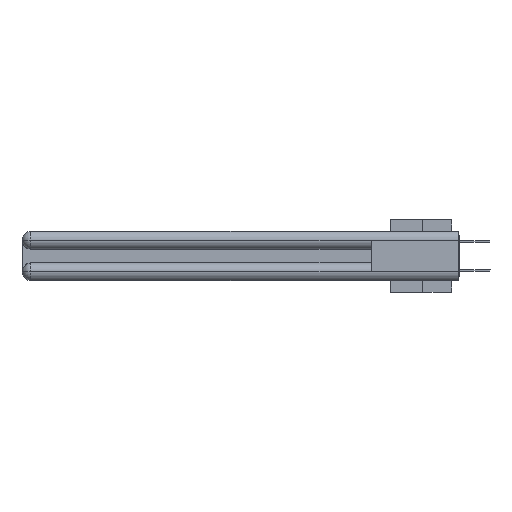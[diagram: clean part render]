
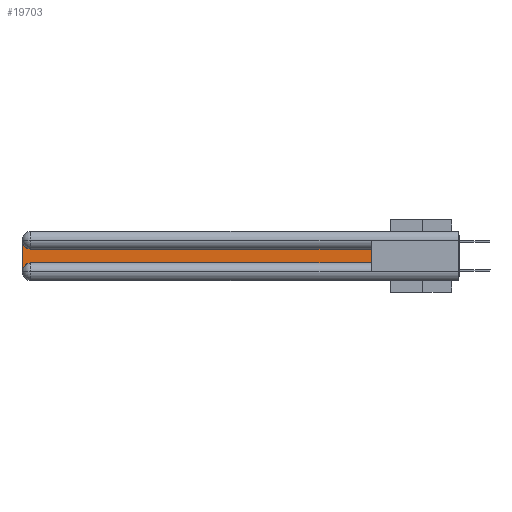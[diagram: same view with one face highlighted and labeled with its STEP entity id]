
A CAD part, left-side view. The second image highlights one B-rep face of the part: STEP entity #19703.
In plain terms, the highlighted planar face has unit normal (-1, 0, 0).
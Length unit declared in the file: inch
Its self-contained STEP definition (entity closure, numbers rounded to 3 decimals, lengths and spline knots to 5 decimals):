
#156 = DIRECTION ( 'NONE',  ( 1., 0., 0. ) ) ;
#2390 = CIRCLE ( 'NONE', #6401, 0.06 ) ;
#2912 = CARTESIAN_POINT ( 'NONE',  ( 0.075, 2.94, -0.0625 ) ) ;
#4606 = CARTESIAN_POINT ( 'NONE',  ( 0.075, 2.94, -0.2775 ) ) ;
#4840 = EDGE_CURVE ( 'NONE', #5301, #26955, #25053, .T. ) ;
#5238 = CARTESIAN_POINT ( 'NONE',  ( 0.075, 3., -0.1225 ) ) ;
#5301 = VERTEX_POINT ( 'NONE', #16665 ) ;
#5591 = AXIS2_PLACEMENT_3D ( 'NONE', #2912, #156, #28526 ) ;
#6158 = VECTOR ( 'NONE', #34325, 39.37008 ) ;
#6401 = AXIS2_PLACEMENT_3D ( 'NONE', #4606, #17427, #30210 ) ;
#6957 = ORIENTED_EDGE ( 'NONE', *, *, #10791, .T. ) ;
#7154 = DIRECTION ( 'NONE',  ( 0., 1., 0. ) ) ;
#7772 = CARTESIAN_POINT ( 'NONE',  ( 0.075, 0.6, -0.1225 ) ) ;
#8352 = CARTESIAN_POINT ( 'NONE',  ( 0.075, 0.6, -0.1225 ) ) ;
#8424 = CARTESIAN_POINT ( 'NONE',  ( 0.075, 2.94, -0.2175 ) ) ;
#8787 = DIRECTION ( 'NONE',  ( 0., 0., 1. ) ) ;
#10519 = LINE ( 'NONE', #7772, #22554 ) ;
#10764 = CARTESIAN_POINT ( 'NONE',  ( 0.075, 0.6, -0.2175 ) ) ;
#10791 = EDGE_CURVE ( 'NONE', #16378, #18903, #31024, .T. ) ;
#11516 = ORIENTED_EDGE ( 'NONE', *, *, #13961, .T. ) ;
#11784 = DIRECTION ( 'NONE',  ( 0., 0., -1. ) ) ;
#12517 = EDGE_LOOP ( 'NONE', ( #29094, #17004, #21422, #11516, #39699, #6957 ) ) ;
#13961 = EDGE_CURVE ( 'NONE', #41506, #39748, #2390, .T. ) ;
#15128 = FACE_OUTER_BOUND ( 'NONE', #12517, .T. ) ;
#16378 = VERTEX_POINT ( 'NONE', #10764 ) ;
#16665 = CARTESIAN_POINT ( 'NONE',  ( 0.075, 2.94, -0.1225 ) ) ;
#16806 = EDGE_CURVE ( 'NONE', #18903, #5301, #10519, .T. ) ;
#17004 = ORIENTED_EDGE ( 'NONE', *, *, #4840, .T. ) ;
#17427 = DIRECTION ( 'NONE',  ( 1., 0., 0. ) ) ;
#17859 = DIRECTION ( 'NONE',  ( 1., 0., 0. ) ) ;
#18283 = LINE ( 'NONE', #24157, #18512 ) ;
#18512 = VECTOR ( 'NONE', #11784, 39.37008 ) ;
#18903 = VERTEX_POINT ( 'NONE', #8352 ) ;
#19703 = ADVANCED_FACE ( 'NONE', ( #15128 ), #30845, .F. ) ;
#20860 = EDGE_CURVE ( 'NONE', #39748, #16378, #41042, .T. ) ;
#21422 = ORIENTED_EDGE ( 'NONE', *, *, #39660, .T. ) ;
#22264 = VECTOR ( 'NONE', #8787, 39.37008 ) ;
#22554 = VECTOR ( 'NONE', #7154, 39.37008 ) ;
#23931 = DIRECTION ( 'NONE',  ( 0., 0., -1. ) ) ;
#24157 = CARTESIAN_POINT ( 'NONE',  ( 0.075, 3., -0.2175 ) ) ;
#25053 = CIRCLE ( 'NONE', #5591, 0.06 ) ;
#26955 = VERTEX_POINT ( 'NONE', #33388 ) ;
#28099 = CARTESIAN_POINT ( 'NONE',  ( 0.075, 0.6, -0.2175 ) ) ;
#28526 = DIRECTION ( 'NONE',  ( 0., 0., -1. ) ) ;
#29094 = ORIENTED_EDGE ( 'NONE', *, *, #16806, .T. ) ;
#30126 = AXIS2_PLACEMENT_3D ( 'NONE', #5238, #17859, #23931 ) ;
#30210 = DIRECTION ( 'NONE',  ( 0., 0., -1. ) ) ;
#30845 = PLANE ( 'NONE',  #30126 ) ;
#31024 = LINE ( 'NONE', #28099, #22264 ) ;
#32041 = CARTESIAN_POINT ( 'NONE',  ( 0.075, 3., -0.2775 ) ) ;
#33388 = CARTESIAN_POINT ( 'NONE',  ( 0.075, 3., -0.0625 ) ) ;
#34325 = DIRECTION ( 'NONE',  ( 0., -1., 0. ) ) ;
#37484 = CARTESIAN_POINT ( 'NONE',  ( 0.075, 0.6, -0.2175 ) ) ;
#39660 = EDGE_CURVE ( 'NONE', #26955, #41506, #18283, .T. ) ;
#39699 = ORIENTED_EDGE ( 'NONE', *, *, #20860, .T. ) ;
#39748 = VERTEX_POINT ( 'NONE', #8424 ) ;
#41042 = LINE ( 'NONE', #37484, #6158 ) ;
#41506 = VERTEX_POINT ( 'NONE', #32041 ) ;
